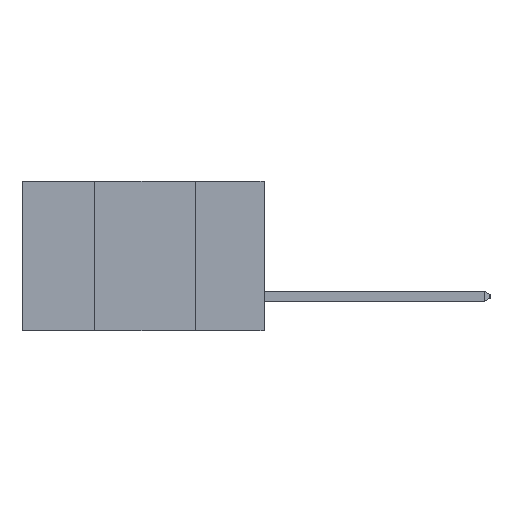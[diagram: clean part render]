
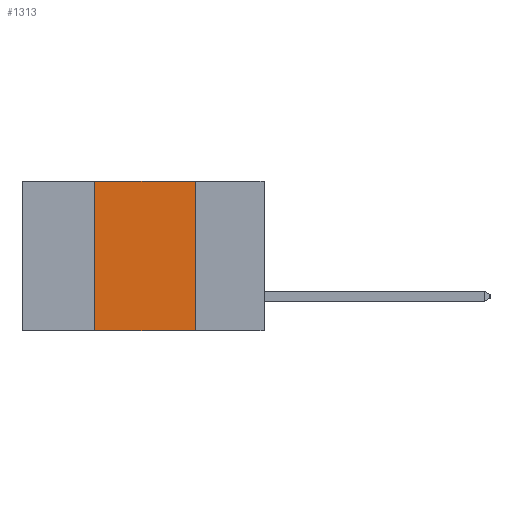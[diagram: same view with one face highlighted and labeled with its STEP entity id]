
A CAD part, left-side view. The second image highlights one B-rep face of the part: STEP entity #1313.
In plain terms, the highlighted planar face has unit normal (-1, 0, 0).
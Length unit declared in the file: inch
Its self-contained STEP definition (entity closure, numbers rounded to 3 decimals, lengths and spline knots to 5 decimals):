
#29 = EDGE_CURVE ( 'NONE', #5295, #16615, #15473, .T. ) ;
#979 = DIRECTION ( 'NONE',  ( 0., -1., 0. ) ) ;
#1144 = DIRECTION ( 'NONE',  ( 0., 0., -1. ) ) ;
#1313 = ADVANCED_FACE ( 'NONE', ( #6667 ), #19772, .F. ) ;
#2567 = VECTOR ( 'NONE', #3663, 39.37008 ) ;
#3487 = CARTESIAN_POINT ( 'NONE',  ( 0., 0.17, -0.37 ) ) ;
#3663 = DIRECTION ( 'NONE',  ( 0., -1., 0. ) ) ;
#4159 = EDGE_CURVE ( 'NONE', #5295, #19639, #17325, .T. ) ;
#4619 = AXIS2_PLACEMENT_3D ( 'NONE', #5104, #7257, #1144 ) ;
#5104 = CARTESIAN_POINT ( 'NONE',  ( 0., 0.6, 0. ) ) ;
#5115 = ORIENTED_EDGE ( 'NONE', *, *, #10115, .F. ) ;
#5295 = VERTEX_POINT ( 'NONE', #23453 ) ;
#6667 = FACE_OUTER_BOUND ( 'NONE', #8500, .T. ) ;
#7257 = DIRECTION ( 'NONE',  ( 1., 0., 0. ) ) ;
#8500 = EDGE_LOOP ( 'NONE', ( #5115, #15490, #20628, #16502 ) ) ;
#9010 = LINE ( 'NONE', #19454, #17700 ) ;
#10115 = EDGE_CURVE ( 'NONE', #20833, #19639, #9010, .T. ) ;
#10137 = CARTESIAN_POINT ( 'NONE',  ( 0., 0.6, 0. ) ) ;
#11089 = VECTOR ( 'NONE', #14697, 39.37008 ) ;
#12845 = CARTESIAN_POINT ( 'NONE',  ( 0., 0.6, -0.37 ) ) ;
#13652 = CARTESIAN_POINT ( 'NONE',  ( 0., 0.17, 0. ) ) ;
#14697 = DIRECTION ( 'NONE',  ( 0., 0., 1. ) ) ;
#14955 = CARTESIAN_POINT ( 'NONE',  ( 0., 0.42, -0.37 ) ) ;
#15473 = LINE ( 'NONE', #14955, #11089 ) ;
#15490 = ORIENTED_EDGE ( 'NONE', *, *, #21559, .F. ) ;
#16297 = CARTESIAN_POINT ( 'NONE',  ( 0., 0.42, 0. ) ) ;
#16502 = ORIENTED_EDGE ( 'NONE', *, *, #4159, .T. ) ;
#16615 = VERTEX_POINT ( 'NONE', #16297 ) ;
#17325 = LINE ( 'NONE', #12845, #2567 ) ;
#17688 = DIRECTION ( 'NONE',  ( 0., 0., -1. ) ) ;
#17700 = VECTOR ( 'NONE', #17688, 39.37008 ) ;
#18825 = VECTOR ( 'NONE', #979, 39.37008 ) ;
#19392 = LINE ( 'NONE', #10137, #18825 ) ;
#19454 = CARTESIAN_POINT ( 'NONE',  ( 0., 0.17, -0.37 ) ) ;
#19639 = VERTEX_POINT ( 'NONE', #3487 ) ;
#19772 = PLANE ( 'NONE',  #4619 ) ;
#20628 = ORIENTED_EDGE ( 'NONE', *, *, #29, .F. ) ;
#20833 = VERTEX_POINT ( 'NONE', #13652 ) ;
#21559 = EDGE_CURVE ( 'NONE', #16615, #20833, #19392, .T. ) ;
#23453 = CARTESIAN_POINT ( 'NONE',  ( 0., 0.42, -0.37 ) ) ;
